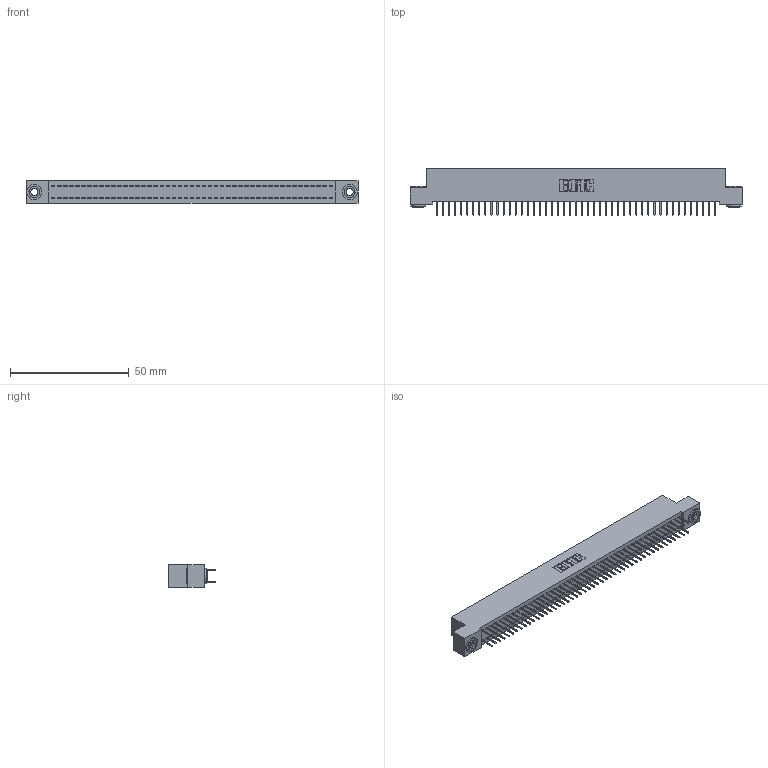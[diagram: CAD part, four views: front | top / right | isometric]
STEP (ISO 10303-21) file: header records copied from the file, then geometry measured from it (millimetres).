
FILE_DESCRIPTION (( 'STEP AP203' ), '1' );
FILE_NAME ('342-094-524-203.STEP', '2019-10-04T15:23:04', ( '' ), ( '' ), 'SwSTEP 2.0', 'SolidWorks 2016', '' );
FILE_SCHEMA (( 'CONFIG_CONTROL_DESIGN' ));
Length unit declared in the file: inch
Products named in the file (4): 342-250-002_345-250-002-102; 342-094-524-203; 342 Part_.156 TH; 345-292-001_345-293-124
Assembly tree (97 placements, depth 2):
  342-094-524-203
    342 Part_.156 TH
    345-292-001_345-293-124  x94
    342-250-002_345-250-002-102  x2
Bounding box: 139.7 x 19.69 x 9.4 mm (x, y, z)
Volume: 12456.3 mm3; surface area: 20242.9 mm2
Topology: 97 solids, 97 shells, 5412 faces, 15321 edges, 9834 vertices
Faces by surface type: plane 4024, cylinder 1380, cone 8
Entity records: 30182 total; most frequent: CARTESIAN_POINT 4969, ORIENTED_EDGE 4898, DIRECTION 4271, EDGE_CURVE 2449, VECTOR 2301, LINE 2301, VERTEX_POINT 1626, AXIS2_PLACEMENT_3D 985
